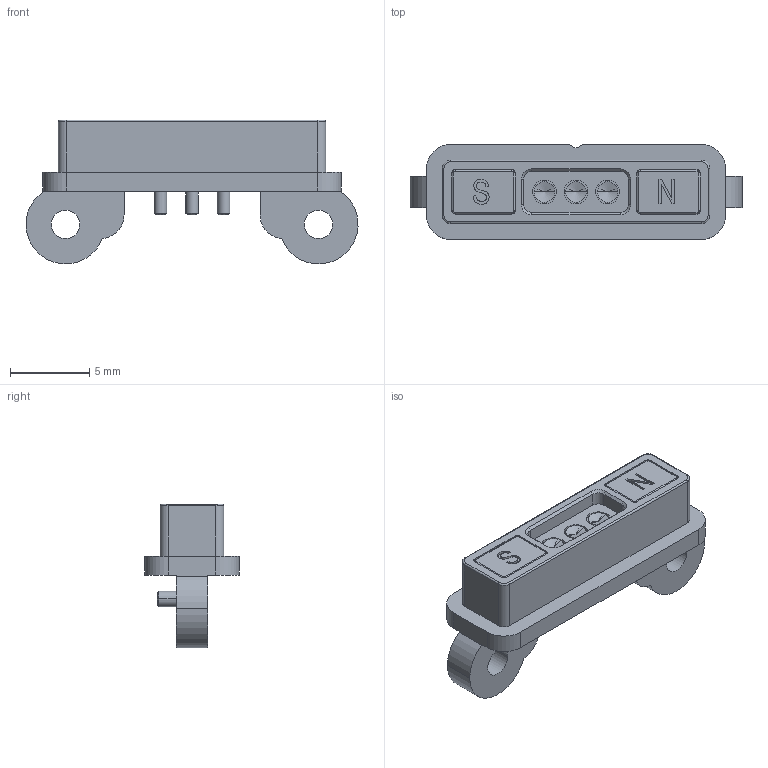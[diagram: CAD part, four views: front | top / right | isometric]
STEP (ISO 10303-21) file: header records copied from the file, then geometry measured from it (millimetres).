
FILE_DESCRIPTION (( 'STEP AP203' ), '1' );
FILE_NAME ('686-F0321250124.STEP', '2023-02-14T10:47:27', ( 'Magnum' ), ( '' ), 'SwSTEP 2.0', 'SolidWorks 2020', '' );
FILE_SCHEMA (( 'CONFIG_CONTROL_DESIGN' ));
Length unit declared in the file: millimetre
Products named in the file (1): 686-F0321250124
Bounding box: 20.99 x 6 x 9.1 mm (x, y, z)
Volume: 395.4 mm3; surface area: 679 mm2
Topology: 4 solids, 6 shells, 239 faces, 569 edges, 354 vertices
Faces by surface type: plane 90, cylinder 88, cone 27, torus 20, bspline 14
Entity records: 7661 total; most frequent: CARTESIAN_POINT 1987, DIRECTION 1208, ORIENTED_EDGE 1126, EDGE_CURVE 563, AXIS2_PLACEMENT_3D 447, VERTEX_POINT 354, VECTOR 314, LINE 314
